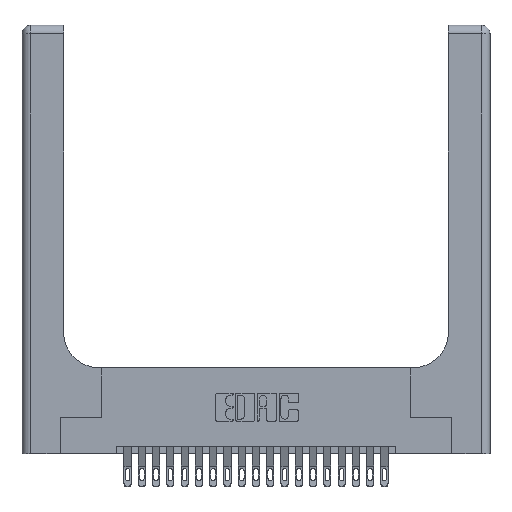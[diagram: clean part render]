
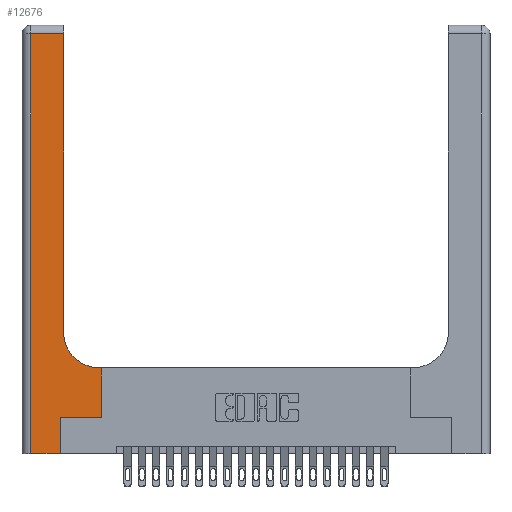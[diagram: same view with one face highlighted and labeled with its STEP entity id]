
A CAD part, top view. The second image highlights one B-rep face of the part: STEP entity #12676.
In plain terms, the highlighted planar face has unit normal (0, 0, 1).
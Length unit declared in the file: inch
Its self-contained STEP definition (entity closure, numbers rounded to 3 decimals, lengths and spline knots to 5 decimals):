
#508 = CARTESIAN_POINT ( 'NONE',  ( 0.5585, 0.6, 0.37 ) ) ;
#600 = ORIENTED_EDGE ( 'NONE', *, *, #6705, .T. ) ;
#644 = EDGE_CURVE ( 'NONE', #16786, #5424, #10706, .T. ) ;
#1258 = CARTESIAN_POINT ( 'NONE',  ( 0.269, 0.25, 0.37 ) ) ;
#1722 = VECTOR ( 'NONE', #10022, 39.37008 ) ;
#1960 = VECTOR ( 'NONE', #18776, 39.37008 ) ;
#2325 = CARTESIAN_POINT ( 'NONE',  ( 0., 3., 0.37 ) ) ;
#2487 = CARTESIAN_POINT ( 'NONE',  ( 0.5415, 0.6, 0.37 ) ) ;
#2560 = ORIENTED_EDGE ( 'NONE', *, *, #4463, .T. ) ;
#2907 = CARTESIAN_POINT ( 'NONE',  ( 0., 2.94, 0.37 ) ) ;
#3385 = ORIENTED_EDGE ( 'NONE', *, *, #5372, .T. ) ;
#3647 = DIRECTION ( 'NONE',  ( 1., 0., 0. ) ) ;
#4124 = CARTESIAN_POINT ( 'NONE',  ( 0.5585, 0.25, 0.37 ) ) ;
#4153 = DIRECTION ( 'NONE',  ( -1., 0., 0. ) ) ;
#4463 = EDGE_CURVE ( 'NONE', #19707, #4504, #20261, .T. ) ;
#4504 = VERTEX_POINT ( 'NONE', #508 ) ;
#4801 = DIRECTION ( 'NONE',  ( -1., 0., 0. ) ) ;
#4835 = AXIS2_PLACEMENT_3D ( 'NONE', #21092, #10145, #22860 ) ;
#5244 = CARTESIAN_POINT ( 'NONE',  ( 0.5585, 0.25, 0.37 ) ) ;
#5312 = VECTOR ( 'NONE', #13365, 39.37008 ) ;
#5372 = EDGE_CURVE ( 'NONE', #23525, #16786, #15491, .T. ) ;
#5374 = ORIENTED_EDGE ( 'NONE', *, *, #6069, .T. ) ;
#5424 = VERTEX_POINT ( 'NONE', #14050 ) ;
#5703 = VECTOR ( 'NONE', #7654, 39.37008 ) ;
#6029 = VECTOR ( 'NONE', #3647, 39.37008 ) ;
#6069 = EDGE_CURVE ( 'NONE', #19601, #19707, #10846, .T. ) ;
#6096 = FACE_OUTER_BOUND ( 'NONE', #15818, .T. ) ;
#6246 = CARTESIAN_POINT ( 'NONE',  ( 0.2915, 0.6, 0.37 ) ) ;
#6705 = EDGE_CURVE ( 'NONE', #9552, #23525, #7938, .T. ) ;
#6988 = EDGE_CURVE ( 'NONE', #13537, #19601, #21671, .T. ) ;
#7397 = VECTOR ( 'NONE', #16596, 39.37008 ) ;
#7654 = DIRECTION ( 'NONE',  ( 0., 1., 0. ) ) ;
#7805 = CARTESIAN_POINT ( 'NONE',  ( 0.2915, 2.94, 0.37 ) ) ;
#7938 = LINE ( 'NONE', #11054, #7397 ) ;
#8038 = EDGE_CURVE ( 'NONE', #5424, #13537, #16499, .T. ) ;
#8918 = ORIENTED_EDGE ( 'NONE', *, *, #8038, .T. ) ;
#9552 = VERTEX_POINT ( 'NONE', #14072 ) ;
#10022 = DIRECTION ( 'NONE',  ( 0., 1., 0. ) ) ;
#10145 = DIRECTION ( 'NONE',  ( 0., 0., -1. ) ) ;
#10613 = VECTOR ( 'NONE', #4801, 39.37008 ) ;
#10706 = LINE ( 'NONE', #13399, #5312 ) ;
#10846 = LINE ( 'NONE', #14576, #6029 ) ;
#10865 = ORIENTED_EDGE ( 'NONE', *, *, #18382, .T. ) ;
#11054 = CARTESIAN_POINT ( 'NONE',  ( 0.2915, 3., 0.37 ) ) ;
#11166 = ORIENTED_EDGE ( 'NONE', *, *, #6988, .T. ) ;
#12676 = ADVANCED_FACE ( 'NONE', ( #6096 ), #13225, .F. ) ;
#13225 = PLANE ( 'NONE',  #18190 ) ;
#13365 = DIRECTION ( 'NONE',  ( 0., -1., 0. ) ) ;
#13399 = CARTESIAN_POINT ( 'NONE',  ( 0.06, 3., 0.37 ) ) ;
#13537 = VERTEX_POINT ( 'NONE', #14165 ) ;
#14050 = CARTESIAN_POINT ( 'NONE',  ( 0.06, 0., 0.37 ) ) ;
#14072 = CARTESIAN_POINT ( 'NONE',  ( 0.2915, 0.85, 0.37 ) ) ;
#14165 = CARTESIAN_POINT ( 'NONE',  ( 0.269, 0., 0.37 ) ) ;
#14524 = VERTEX_POINT ( 'NONE', #2487 ) ;
#14576 = CARTESIAN_POINT ( 'NONE',  ( 0.269, 0.25, 0.37 ) ) ;
#14759 = LINE ( 'NONE', #6246, #19029 ) ;
#15084 = DIRECTION ( 'NONE',  ( 0., 0., -1. ) ) ;
#15199 = CARTESIAN_POINT ( 'NONE',  ( 0., 0., 0.37 ) ) ;
#15491 = LINE ( 'NONE', #2907, #10613 ) ;
#15818 = EDGE_LOOP ( 'NONE', ( #600, #3385, #19032, #8918, #11166, #5374, #2560, #19615, #10865 ) ) ;
#16499 = LINE ( 'NONE', #15199, #1960 ) ;
#16596 = DIRECTION ( 'NONE',  ( 0., 1., 0. ) ) ;
#16786 = VERTEX_POINT ( 'NONE', #21791 ) ;
#18190 = AXIS2_PLACEMENT_3D ( 'NONE', #2325, #15084, #4153 ) ;
#18382 = EDGE_CURVE ( 'NONE', #14524, #9552, #22486, .T. ) ;
#18776 = DIRECTION ( 'NONE',  ( 1., 0., 0. ) ) ;
#19029 = VECTOR ( 'NONE', #20849, 39.37008 ) ;
#19032 = ORIENTED_EDGE ( 'NONE', *, *, #644, .T. ) ;
#19601 = VERTEX_POINT ( 'NONE', #1258 ) ;
#19615 = ORIENTED_EDGE ( 'NONE', *, *, #20050, .T. ) ;
#19707 = VERTEX_POINT ( 'NONE', #5244 ) ;
#20050 = EDGE_CURVE ( 'NONE', #4504, #14524, #14759, .T. ) ;
#20261 = LINE ( 'NONE', #4124, #5703 ) ;
#20849 = DIRECTION ( 'NONE',  ( -1., 0., 0. ) ) ;
#20959 = CARTESIAN_POINT ( 'NONE',  ( 0.269, 0., 0.37 ) ) ;
#21092 = CARTESIAN_POINT ( 'NONE',  ( 0.5415, 0.85, 0.37 ) ) ;
#21671 = LINE ( 'NONE', #20959, #1722 ) ;
#21791 = CARTESIAN_POINT ( 'NONE',  ( 0.06, 2.94, 0.37 ) ) ;
#22486 = CIRCLE ( 'NONE', #4835, 0.25 ) ;
#22860 = DIRECTION ( 'NONE',  ( 1., 0., 0. ) ) ;
#23525 = VERTEX_POINT ( 'NONE', #7805 ) ;
